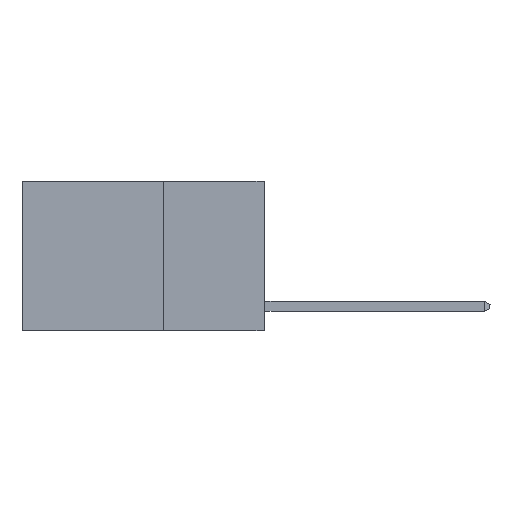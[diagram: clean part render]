
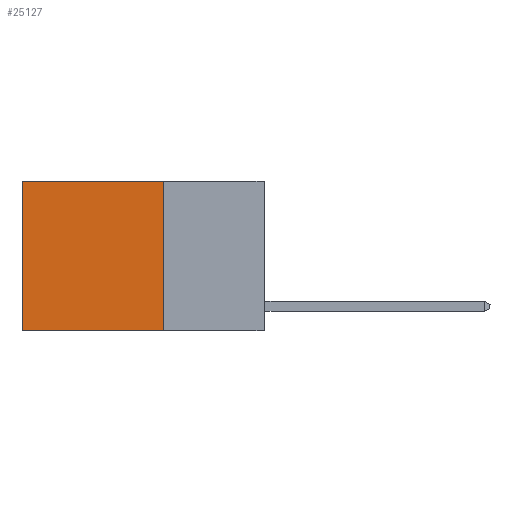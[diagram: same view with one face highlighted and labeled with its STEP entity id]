
A CAD part, left-side view. The second image highlights one B-rep face of the part: STEP entity #25127.
In plain terms, the highlighted planar face has unit normal (-1, 0, 0).
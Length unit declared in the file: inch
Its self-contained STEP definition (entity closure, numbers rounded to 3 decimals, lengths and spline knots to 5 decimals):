
#904 = LINE ( 'NONE', #18403, #12585 ) ;
#1133 = DIRECTION ( 'NONE',  ( 0., 0., -1. ) ) ;
#1221 = LINE ( 'NONE', #25262, #19136 ) ;
#1509 = VECTOR ( 'NONE', #1133, 39.37008 ) ;
#3533 = VERTEX_POINT ( 'NONE', #14799 ) ;
#3773 = ORIENTED_EDGE ( 'NONE', *, *, #22753, .F. ) ;
#4379 = DIRECTION ( 'NONE',  ( 0., 1., 0. ) ) ;
#6778 = DIRECTION ( 'NONE',  ( 0., 1., 0. ) ) ;
#6917 = EDGE_CURVE ( 'NONE', #19801, #19813, #9981, .T. ) ;
#8287 = EDGE_LOOP ( 'NONE', ( #9252, #3773, #18710, #10891 ) ) ;
#8581 = DIRECTION ( 'NONE',  ( 0., 0., -1. ) ) ;
#9252 = ORIENTED_EDGE ( 'NONE', *, *, #6917, .T. ) ;
#9981 = LINE ( 'NONE', #13220, #16182 ) ;
#10426 = CARTESIAN_POINT ( 'NONE',  ( 0.2625, 0.25, 0. ) ) ;
#10814 = CARTESIAN_POINT ( 'NONE',  ( 0.2625, 0.25, 0. ) ) ;
#10891 = ORIENTED_EDGE ( 'NONE', *, *, #23377, .T. ) ;
#11366 = CARTESIAN_POINT ( 'NONE',  ( 0.2625, 0.25, 0. ) ) ;
#11548 = CARTESIAN_POINT ( 'NONE',  ( 0.2625, 0.6, 0. ) ) ;
#12585 = VECTOR ( 'NONE', #6778, 39.37008 ) ;
#13220 = CARTESIAN_POINT ( 'NONE',  ( 0.2625, 0.6, 0. ) ) ;
#14799 = CARTESIAN_POINT ( 'NONE',  ( 0.2625, 0.25, -0.37 ) ) ;
#16182 = VECTOR ( 'NONE', #29469, 39.37008 ) ;
#17869 = PLANE ( 'NONE',  #25314 ) ;
#18403 = CARTESIAN_POINT ( 'NONE',  ( 0.2625, 0.25, -0.37 ) ) ;
#18710 = ORIENTED_EDGE ( 'NONE', *, *, #24447, .F. ) ;
#19136 = VECTOR ( 'NONE', #4379, 39.37008 ) ;
#19801 = VERTEX_POINT ( 'NONE', #11548 ) ;
#19813 = VERTEX_POINT ( 'NONE', #20964 ) ;
#20142 = LINE ( 'NONE', #10426, #1509 ) ;
#20964 = CARTESIAN_POINT ( 'NONE',  ( 0.2625, 0.6, -0.37 ) ) ;
#22555 = DIRECTION ( 'NONE',  ( 1., 0., 0. ) ) ;
#22753 = EDGE_CURVE ( 'NONE', #3533, #19813, #904, .T. ) ;
#23377 = EDGE_CURVE ( 'NONE', #25923, #19801, #1221, .T. ) ;
#24447 = EDGE_CURVE ( 'NONE', #25923, #3533, #20142, .T. ) ;
#24458 = FACE_OUTER_BOUND ( 'NONE', #8287, .T. ) ;
#25127 = ADVANCED_FACE ( 'NONE', ( #24458 ), #17869, .F. ) ;
#25262 = CARTESIAN_POINT ( 'NONE',  ( 0.2625, 0.25, 0. ) ) ;
#25314 = AXIS2_PLACEMENT_3D ( 'NONE', #10814, #22555, #8581 ) ;
#25923 = VERTEX_POINT ( 'NONE', #11366 ) ;
#29469 = DIRECTION ( 'NONE',  ( 0., 0., -1. ) ) ;
